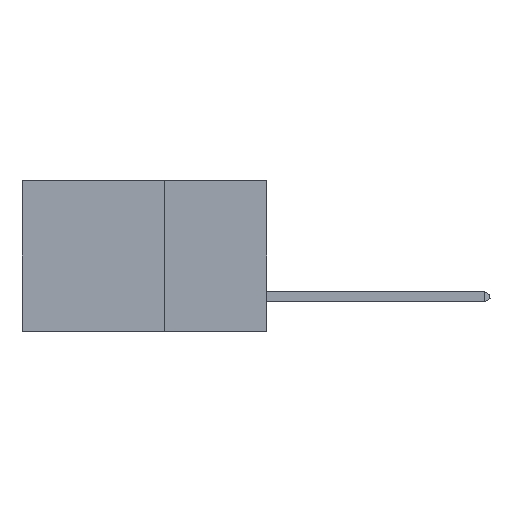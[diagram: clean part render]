
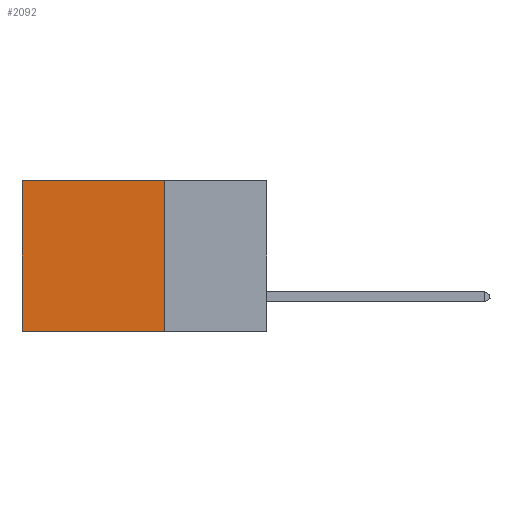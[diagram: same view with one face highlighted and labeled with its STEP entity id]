
A CAD part, left-side view. The second image highlights one B-rep face of the part: STEP entity #2092.
In plain terms, the highlighted planar face has unit normal (-1, 0, 0).
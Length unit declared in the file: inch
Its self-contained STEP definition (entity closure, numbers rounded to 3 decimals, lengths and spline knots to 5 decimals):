
#88 = VERTEX_POINT ( 'NONE', #12537 ) ;
#595 = DIRECTION ( 'NONE',  ( 1., 0., 0. ) ) ;
#802 = PLANE ( 'NONE',  #11525 ) ;
#804 = LINE ( 'NONE', #18509, #1623 ) ;
#1623 = VECTOR ( 'NONE', #15417, 39.37008 ) ;
#2092 = ADVANCED_FACE ( 'NONE', ( #6647 ), #802, .F. ) ;
#2389 = DIRECTION ( 'NONE',  ( 0., 0., -1. ) ) ;
#2658 = EDGE_CURVE ( 'NONE', #20862, #4894, #804, .T. ) ;
#2908 = CARTESIAN_POINT ( 'NONE',  ( 0.2875, 0.6, 0. ) ) ;
#3148 = EDGE_CURVE ( 'NONE', #4894, #88, #6449, .T. ) ;
#3610 = CARTESIAN_POINT ( 'NONE',  ( 0.2875, 0.25, -0.37 ) ) ;
#3960 = DIRECTION ( 'NONE',  ( 0., 0., -1. ) ) ;
#4679 = ORIENTED_EDGE ( 'NONE', *, *, #3148, .T. ) ;
#4894 = VERTEX_POINT ( 'NONE', #2908 ) ;
#6053 = ORIENTED_EDGE ( 'NONE', *, *, #2658, .T. ) ;
#6312 = VECTOR ( 'NONE', #20137, 39.37008 ) ;
#6449 = LINE ( 'NONE', #15708, #13049 ) ;
#6647 = FACE_OUTER_BOUND ( 'NONE', #13322, .T. ) ;
#9100 = VECTOR ( 'NONE', #2389, 39.37008 ) ;
#9593 = ORIENTED_EDGE ( 'NONE', *, *, #11031, .F. ) ;
#10605 = CARTESIAN_POINT ( 'NONE',  ( 0.2875, 0.25, 0. ) ) ;
#10789 = LINE ( 'NONE', #11889, #6312 ) ;
#11031 = EDGE_CURVE ( 'NONE', #20862, #16682, #18557, .T. ) ;
#11525 = AXIS2_PLACEMENT_3D ( 'NONE', #12292, #595, #3960 ) ;
#11889 = CARTESIAN_POINT ( 'NONE',  ( 0.2875, 0.25, -0.37 ) ) ;
#12292 = CARTESIAN_POINT ( 'NONE',  ( 0.2875, 0.25, 0. ) ) ;
#12344 = CARTESIAN_POINT ( 'NONE',  ( 0.2875, 0.25, 0. ) ) ;
#12537 = CARTESIAN_POINT ( 'NONE',  ( 0.2875, 0.6, -0.37 ) ) ;
#13049 = VECTOR ( 'NONE', #18938, 39.37008 ) ;
#13319 = ORIENTED_EDGE ( 'NONE', *, *, #16344, .F. ) ;
#13322 = EDGE_LOOP ( 'NONE', ( #4679, #13319, #9593, #6053 ) ) ;
#15417 = DIRECTION ( 'NONE',  ( 0., 1., 0. ) ) ;
#15708 = CARTESIAN_POINT ( 'NONE',  ( 0.2875, 0.6, 0. ) ) ;
#16344 = EDGE_CURVE ( 'NONE', #16682, #88, #10789, .T. ) ;
#16682 = VERTEX_POINT ( 'NONE', #3610 ) ;
#18509 = CARTESIAN_POINT ( 'NONE',  ( 0.2875, 0.25, 0. ) ) ;
#18557 = LINE ( 'NONE', #12344, #9100 ) ;
#18938 = DIRECTION ( 'NONE',  ( 0., 0., -1. ) ) ;
#20137 = DIRECTION ( 'NONE',  ( 0., 1., 0. ) ) ;
#20862 = VERTEX_POINT ( 'NONE', #10605 ) ;
